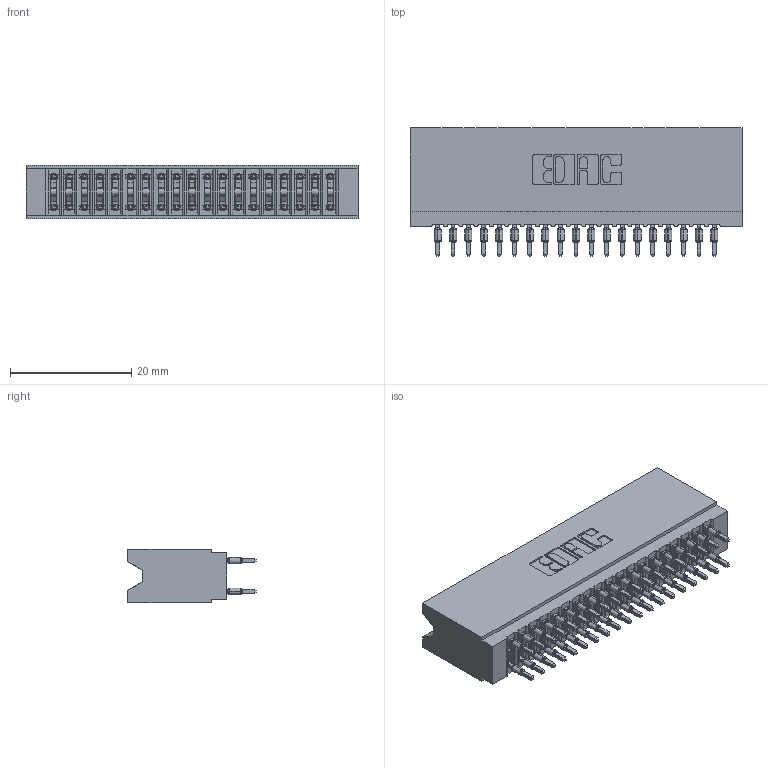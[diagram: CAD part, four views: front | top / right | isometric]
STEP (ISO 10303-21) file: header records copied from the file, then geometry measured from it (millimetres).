
FILE_DESCRIPTION (( 'STEP AP203' ), '1' );
FILE_NAME ('745-038-560-206.STEP', '2026-02-26T17:30:02', ( '' ), ( '' ), 'SwSTEP 2.0', 'SolidWorks 2023', '' );
FILE_SCHEMA (( 'CONFIG_CONTROL_DESIGN' ));
Length unit declared in the file: millimetre
Products named in the file (3): 745 Part_Insulator Option - 06; 745-038-560-206; 745-292-001_560
Assembly tree (39 placements, depth 2):
  745-038-560-206
    745 Part_Insulator Option - 06
    745-292-001_560  x38
Bounding box: 54.86 x 21.22 x 8.89 mm (x, y, z)
Volume: 5198 mm3; surface area: 10661.2 mm2
Topology: 39 solids, 39 shells, 3839 faces, 10501 edges, 6670 vertices
Faces by surface type: plane 1994, cylinder 857, bspline 760, torus 228
Entity records: 35470 total; most frequent: CARTESIAN_POINT 6664, ORIENTED_EDGE 6054, DIRECTION 5313, EDGE_CURVE 3027, LINE 2723, VECTOR 2723, VERTEX_POINT 1934, AXIS2_PLACEMENT_3D 1295
